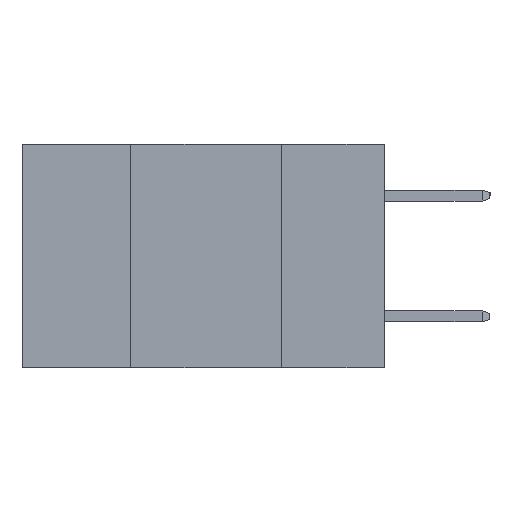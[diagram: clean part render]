
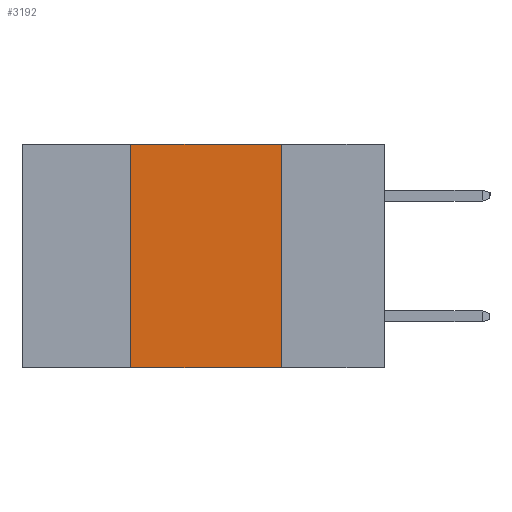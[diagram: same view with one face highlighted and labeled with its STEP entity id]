
A CAD part, left-side view. The second image highlights one B-rep face of the part: STEP entity #3192.
In plain terms, the highlighted planar face has unit normal (-1, 0, 0).
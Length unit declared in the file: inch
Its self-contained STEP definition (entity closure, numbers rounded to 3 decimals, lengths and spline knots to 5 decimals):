
#786 = CARTESIAN_POINT ( 'NONE',  ( 0., 0.42, 0. ) ) ;
#1573 = VERTEX_POINT ( 'NONE', #11570 ) ;
#3192 = ADVANCED_FACE ( 'NONE', ( #5923 ), #7938, .F. ) ;
#3496 = ORIENTED_EDGE ( 'NONE', *, *, #15631, .F. ) ;
#3527 = ORIENTED_EDGE ( 'NONE', *, *, #4578, .F. ) ;
#3678 = CARTESIAN_POINT ( 'NONE',  ( 0., 0.6, 0. ) ) ;
#4495 = ORIENTED_EDGE ( 'NONE', *, *, #10465, .T. ) ;
#4578 = EDGE_CURVE ( 'NONE', #7970, #10934, #11805, .T. ) ;
#5061 = CARTESIAN_POINT ( 'NONE',  ( 0., 0.17, -0.37 ) ) ;
#5923 = FACE_OUTER_BOUND ( 'NONE', #15228, .T. ) ;
#6243 = ORIENTED_EDGE ( 'NONE', *, *, #8744, .F. ) ;
#6624 = CARTESIAN_POINT ( 'NONE',  ( 0., 0.42, -0.37 ) ) ;
#6730 = DIRECTION ( 'NONE',  ( 1., 0., 0. ) ) ;
#6824 = CARTESIAN_POINT ( 'NONE',  ( 0., 0.17, 0. ) ) ;
#7938 = PLANE ( 'NONE',  #16605 ) ;
#7970 = VERTEX_POINT ( 'NONE', #6824 ) ;
#8111 = CARTESIAN_POINT ( 'NONE',  ( 0., 0.6, 0. ) ) ;
#8697 = LINE ( 'NONE', #15164, #14693 ) ;
#8744 = EDGE_CURVE ( 'NONE', #15400, #7970, #16841, .T. ) ;
#8978 = DIRECTION ( 'NONE',  ( 0., -1., 0. ) ) ;
#9780 = VECTOR ( 'NONE', #10763, 39.37008 ) ;
#10062 = DIRECTION ( 'NONE',  ( 0., -1., 0. ) ) ;
#10465 = EDGE_CURVE ( 'NONE', #1573, #10934, #8697, .T. ) ;
#10666 = DIRECTION ( 'NONE',  ( 0., 0., -1. ) ) ;
#10763 = DIRECTION ( 'NONE',  ( 0., 0., 1. ) ) ;
#10934 = VERTEX_POINT ( 'NONE', #5061 ) ;
#11570 = CARTESIAN_POINT ( 'NONE',  ( 0., 0.42, -0.37 ) ) ;
#11805 = LINE ( 'NONE', #15625, #16845 ) ;
#12704 = VECTOR ( 'NONE', #8978, 39.37008 ) ;
#14518 = DIRECTION ( 'NONE',  ( 0., 0., -1. ) ) ;
#14693 = VECTOR ( 'NONE', #10062, 39.37008 ) ;
#15164 = CARTESIAN_POINT ( 'NONE',  ( 0., 0.6, -0.37 ) ) ;
#15228 = EDGE_LOOP ( 'NONE', ( #3527, #6243, #3496, #4495 ) ) ;
#15400 = VERTEX_POINT ( 'NONE', #786 ) ;
#15625 = CARTESIAN_POINT ( 'NONE',  ( 0., 0.17, -0.37 ) ) ;
#15631 = EDGE_CURVE ( 'NONE', #1573, #15400, #17102, .T. ) ;
#16605 = AXIS2_PLACEMENT_3D ( 'NONE', #8111, #6730, #14518 ) ;
#16841 = LINE ( 'NONE', #3678, #12704 ) ;
#16845 = VECTOR ( 'NONE', #10666, 39.37008 ) ;
#17102 = LINE ( 'NONE', #6624, #9780 ) ;
